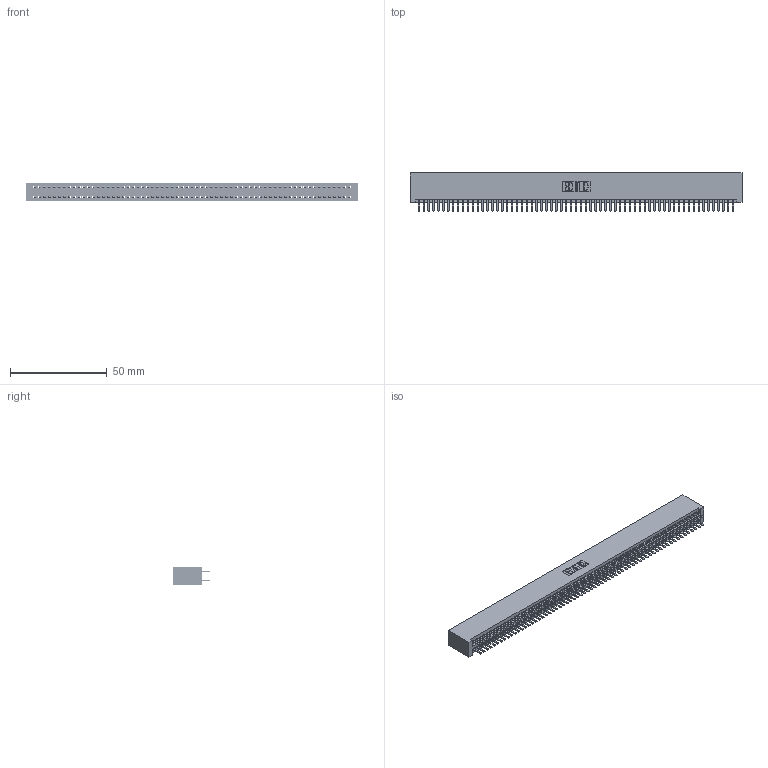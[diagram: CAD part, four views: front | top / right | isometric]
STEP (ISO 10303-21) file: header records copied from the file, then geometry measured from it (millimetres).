
FILE_DESCRIPTION (( 'STEP AP203' ), '1' );
FILE_NAME ('345-130-520-201.STEP', '2019-11-07T11:48:56', ( '' ), ( '' ), 'SwSTEP 2.0', 'SolidWorks 2016', '' );
FILE_SCHEMA (( 'CONFIG_CONTROL_DESIGN' ));
Length unit declared in the file: inch
Products named in the file (3): 345 Part_No Mounting Lugs; 345-130-520-201; 345-292-001_345-293-120
Assembly tree (131 placements, depth 2):
  345-130-520-201
    345 Part_No Mounting Lugs
    345-292-001_345-293-120  x130
Bounding box: 171.7 x 19.68 x 9.4 mm (x, y, z)
Volume: 17451.8 mm3; surface area: 26423.8 mm2
Topology: 131 solids, 131 shells, 7138 faces, 20727 edges, 13470 vertices
Faces by surface type: plane 4626, cylinder 2512
Entity records: 47741 total; most frequent: CARTESIAN_POINT 7992, ORIENTED_EDGE 7914, DIRECTION 7001, EDGE_CURVE 3957, VECTOR 3569, LINE 3569, VERTEX_POINT 2634, AXIS2_PLACEMENT_3D 1716
